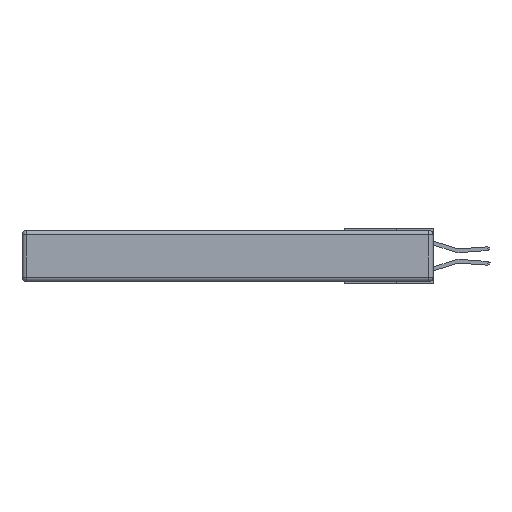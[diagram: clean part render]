
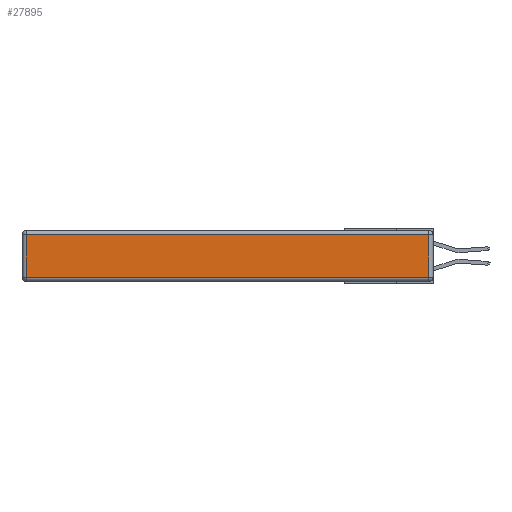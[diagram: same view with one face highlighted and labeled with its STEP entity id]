
A CAD part, left-side view. The second image highlights one B-rep face of the part: STEP entity #27895.
In plain terms, the highlighted planar face has unit normal (-1, 0, 0).
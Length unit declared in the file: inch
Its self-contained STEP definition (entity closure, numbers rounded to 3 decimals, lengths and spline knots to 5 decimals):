
#1137 = VERTEX_POINT ( 'NONE', #2141 ) ;
#1911 = VECTOR ( 'NONE', #6054, 39.37008 ) ;
#2141 = CARTESIAN_POINT ( 'NONE',  ( 0., 2.72, -0.03 ) ) ;
#3221 = DIRECTION ( 'NONE',  ( -1., 0., 0. ) ) ;
#3406 = DIRECTION ( 'NONE',  ( 0., 0., 1. ) ) ;
#4406 = VERTEX_POINT ( 'NONE', #9386 ) ;
#4608 = ORIENTED_EDGE ( 'NONE', *, *, #25865, .T. ) ;
#5850 = DIRECTION ( 'NONE',  ( 0., 0., 1. ) ) ;
#6054 = DIRECTION ( 'NONE',  ( 0., -1., 0. ) ) ;
#6451 = VECTOR ( 'NONE', #24987, 39.37008 ) ;
#7639 = CARTESIAN_POINT ( 'NONE',  ( 0., 0., -0.343 ) ) ;
#7766 = DIRECTION ( 'NONE',  ( 0., 0., -1. ) ) ;
#7899 = VECTOR ( 'NONE', #5850, 39.37008 ) ;
#8883 = LINE ( 'NONE', #23081, #6451 ) ;
#9386 = CARTESIAN_POINT ( 'NONE',  ( 0., 2.72, -0.313 ) ) ;
#9845 = EDGE_LOOP ( 'NONE', ( #25393, #4608, #14147, #19799 ) ) ;
#10453 = EDGE_CURVE ( 'NONE', #12876, #1137, #8883, .T. ) ;
#11286 = EDGE_CURVE ( 'NONE', #4406, #25474, #26567, .T. ) ;
#12876 = VERTEX_POINT ( 'NONE', #17731 ) ;
#13406 = FACE_OUTER_BOUND ( 'NONE', #9845, .T. ) ;
#14147 = ORIENTED_EDGE ( 'NONE', *, *, #10453, .T. ) ;
#14463 = CARTESIAN_POINT ( 'NONE',  ( 0., 2.72, -0.343 ) ) ;
#14526 = PLANE ( 'NONE',  #24149 ) ;
#16081 = EDGE_CURVE ( 'NONE', #1137, #4406, #16367, .T. ) ;
#16367 = LINE ( 'NONE', #14463, #18757 ) ;
#17731 = CARTESIAN_POINT ( 'NONE',  ( 0., 0.03, -0.03 ) ) ;
#18757 = VECTOR ( 'NONE', #7766, 39.37008 ) ;
#19400 = CARTESIAN_POINT ( 'NONE',  ( 0., 0.03, -0.313 ) ) ;
#19799 = ORIENTED_EDGE ( 'NONE', *, *, #16081, .T. ) ;
#21361 = CARTESIAN_POINT ( 'NONE',  ( 0., 0.03, -0.343 ) ) ;
#23081 = CARTESIAN_POINT ( 'NONE',  ( 0., 2.75, -0.03 ) ) ;
#24149 = AXIS2_PLACEMENT_3D ( 'NONE', #7639, #3221, #3406 ) ;
#24987 = DIRECTION ( 'NONE',  ( 0., 1., 0. ) ) ;
#25318 = LINE ( 'NONE', #21361, #7899 ) ;
#25393 = ORIENTED_EDGE ( 'NONE', *, *, #11286, .T. ) ;
#25474 = VERTEX_POINT ( 'NONE', #19400 ) ;
#25657 = CARTESIAN_POINT ( 'NONE',  ( 0., 0., -0.313 ) ) ;
#25865 = EDGE_CURVE ( 'NONE', #25474, #12876, #25318, .T. ) ;
#26567 = LINE ( 'NONE', #25657, #1911 ) ;
#27895 = ADVANCED_FACE ( 'NONE', ( #13406 ), #14526, .T. ) ;
